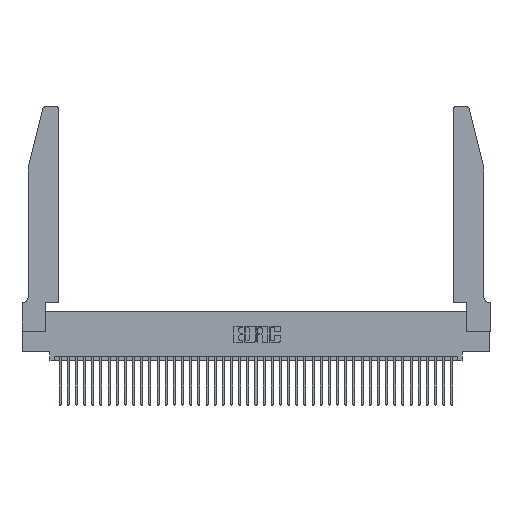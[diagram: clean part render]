
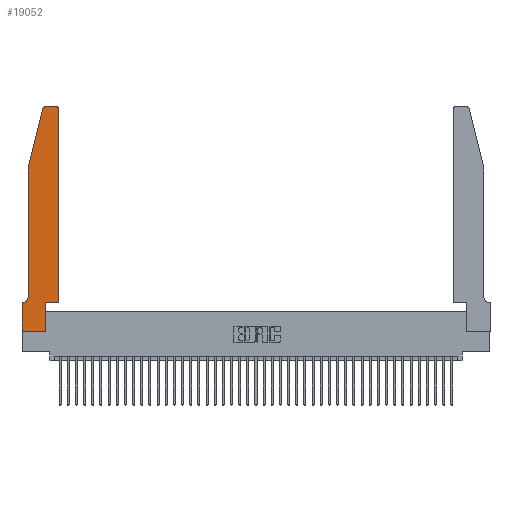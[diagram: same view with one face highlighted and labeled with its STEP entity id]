
A CAD part, top view. The second image highlights one B-rep face of the part: STEP entity #19052.
In plain terms, the highlighted planar face has unit normal (0, 0, 1).
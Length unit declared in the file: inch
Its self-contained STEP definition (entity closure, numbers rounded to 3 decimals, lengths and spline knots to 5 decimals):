
#363 = VECTOR ( 'NONE', #24415, 39.37008 ) ;
#1024 = AXIS2_PLACEMENT_3D ( 'NONE', #33563, #13965, #36864 ) ;
#1326 = VERTEX_POINT ( 'NONE', #29959 ) ;
#2813 = DIRECTION ( 'NONE',  ( 0., -1., 0. ) ) ;
#2863 = VECTOR ( 'NONE', #3584, 39.37008 ) ;
#3584 = DIRECTION ( 'NONE',  ( 1., 0., 0. ) ) ;
#4848 = CARTESIAN_POINT ( 'NONE',  ( 0.25487, 2.72718, 0.37 ) ) ;
#5324 = CIRCLE ( 'NONE', #18917, 0.03 ) ;
#5350 = LINE ( 'NONE', #19186, #13074 ) ;
#6082 = VERTEX_POINT ( 'NONE', #38138 ) ;
#6391 = PLANE ( 'NONE',  #8394 ) ;
#6947 = CIRCLE ( 'NONE', #11738, 0.07 ) ;
#7452 = VERTEX_POINT ( 'NONE', #22876 ) ;
#7635 = CARTESIAN_POINT ( 'NONE',  ( 0.4505, 0.35, 0.37 ) ) ;
#7849 = DIRECTION ( 'NONE',  ( 1., 0., 0. ) ) ;
#8078 = EDGE_CURVE ( 'NONE', #39810, #19090, #25536, .T. ) ;
#8394 = AXIS2_PLACEMENT_3D ( 'NONE', #29358, #42300, #32603 ) ;
#9282 = CARTESIAN_POINT ( 'NONE',  ( 0., 0.35, 0.37 ) ) ;
#10536 = CARTESIAN_POINT ( 'NONE',  ( 0., 0., 0.37 ) ) ;
#10678 = CARTESIAN_POINT ( 'NONE',  ( 0.284, 2.72, 0.37 ) ) ;
#11385 = CARTESIAN_POINT ( 'NONE',  ( 0.2865, 0.35, 0.37 ) ) ;
#11691 = ORIENTED_EDGE ( 'NONE', *, *, #30988, .T. ) ;
#11738 = AXIS2_PLACEMENT_3D ( 'NONE', #36510, #16945, #39782 ) ;
#11981 = CARTESIAN_POINT ( 'NONE',  ( 0.2605, 2.75, 0.37 ) ) ;
#12430 = ORIENTED_EDGE ( 'NONE', *, *, #36081, .T. ) ;
#13074 = VECTOR ( 'NONE', #2813, 39.37008 ) ;
#13147 = CARTESIAN_POINT ( 'NONE',  ( 0.2865, 0.35, 0.37 ) ) ;
#13965 = DIRECTION ( 'NONE',  ( 0., 0., 1. ) ) ;
#13988 = DIRECTION ( 'NONE',  ( 1., 0., 0. ) ) ;
#15048 = DIRECTION ( 'NONE',  ( -0.239, -0.971, 0. ) ) ;
#15246 = VECTOR ( 'NONE', #20415, 39.37008 ) ;
#15438 = VECTOR ( 'NONE', #25013, 39.37008 ) ;
#16472 = LINE ( 'NONE', #11981, #15438 ) ;
#16945 = DIRECTION ( 'NONE',  ( 0., 0., -1. ) ) ;
#16980 = EDGE_CURVE ( 'NONE', #7452, #6082, #5350, .T. ) ;
#17027 = EDGE_LOOP ( 'NONE', ( #11691, #37344, #27750, #29146, #17499, #17978, #35361, #12430, #35993, #18125, #27890, #22286 ) ) ;
#17499 = ORIENTED_EDGE ( 'NONE', *, *, #34721, .T. ) ;
#17978 = ORIENTED_EDGE ( 'NONE', *, *, #35241, .T. ) ;
#18125 = ORIENTED_EDGE ( 'NONE', *, *, #21626, .T. ) ;
#18326 = LINE ( 'NONE', #10536, #15246 ) ;
#18813 = EDGE_CURVE ( 'NONE', #36352, #7452, #26732, .T. ) ;
#18917 = AXIS2_PLACEMENT_3D ( 'NONE', #10678, #33585, #13988 ) ;
#19052 = ADVANCED_FACE ( 'NONE', ( #19534 ), #6391, .T. ) ;
#19090 = VERTEX_POINT ( 'NONE', #13147 ) ;
#19186 = CARTESIAN_POINT ( 'NONE',  ( 0.0755, 2., 0.37 ) ) ;
#19284 = CARTESIAN_POINT ( 'NONE',  ( 0.4205, 2.75, 0.37 ) ) ;
#19534 = FACE_OUTER_BOUND ( 'NONE', #17027, .T. ) ;
#20415 = DIRECTION ( 'NONE',  ( 0., -1., 0. ) ) ;
#21626 = EDGE_CURVE ( 'NONE', #19090, #39589, #35754, .T. ) ;
#22187 = EDGE_CURVE ( 'NONE', #1326, #37210, #32626, .T. ) ;
#22286 = ORIENTED_EDGE ( 'NONE', *, *, #22187, .T. ) ;
#22876 = CARTESIAN_POINT ( 'NONE',  ( 0.0755, 2., 0.37 ) ) ;
#24415 = DIRECTION ( 'NONE',  ( 0., 1., 0. ) ) ;
#25013 = DIRECTION ( 'NONE',  ( -1., 0., 0. ) ) ;
#25536 = LINE ( 'NONE', #11385, #363 ) ;
#25884 = CARTESIAN_POINT ( 'NONE',  ( 0.0755, 0.35, 0.37 ) ) ;
#25982 = CARTESIAN_POINT ( 'NONE',  ( 0., 0., 0.37 ) ) ;
#26484 = VERTEX_POINT ( 'NONE', #32318 ) ;
#26544 = CARTESIAN_POINT ( 'NONE',  ( 0., 0., 0.37 ) ) ;
#26732 = LINE ( 'NONE', #34632, #35424 ) ;
#27085 = VECTOR ( 'NONE', #7849, 39.37008 ) ;
#27470 = CARTESIAN_POINT ( 'NONE',  ( 0.4505, 0.35, 0.37 ) ) ;
#27526 = CARTESIAN_POINT ( 'NONE',  ( 0.2865, 0., 0.37 ) ) ;
#27540 = DIRECTION ( 'NONE',  ( 0., 1., 0. ) ) ;
#27750 = ORIENTED_EDGE ( 'NONE', *, *, #18813, .T. ) ;
#27890 = ORIENTED_EDGE ( 'NONE', *, *, #32850, .T. ) ;
#29146 = ORIENTED_EDGE ( 'NONE', *, *, #16980, .T. ) ;
#29210 = DIRECTION ( 'NONE',  ( -1., 0., 0. ) ) ;
#29358 = CARTESIAN_POINT ( 'NONE',  ( 0., 0.35, 0.37 ) ) ;
#29708 = CARTESIAN_POINT ( 'NONE',  ( 0.4505, 0.35, 0.37 ) ) ;
#29959 = CARTESIAN_POINT ( 'NONE',  ( 0.4505, 2.72, 0.37 ) ) ;
#30988 = EDGE_CURVE ( 'NONE', #37210, #26484, #16472, .T. ) ;
#31012 = VECTOR ( 'NONE', #29210, 39.37008 ) ;
#31095 = VERTEX_POINT ( 'NONE', #9282 ) ;
#32318 = CARTESIAN_POINT ( 'NONE',  ( 0.284, 2.75, 0.37 ) ) ;
#32603 = DIRECTION ( 'NONE',  ( 1., 0., 0. ) ) ;
#32626 = CIRCLE ( 'NONE', #1024, 0.03 ) ;
#32661 = VECTOR ( 'NONE', #27540, 39.37008 ) ;
#32850 = EDGE_CURVE ( 'NONE', #39589, #1326, #33695, .T. ) ;
#33563 = CARTESIAN_POINT ( 'NONE',  ( 0.4205, 2.72, 0.37 ) ) ;
#33585 = DIRECTION ( 'NONE',  ( 0., 0., 1. ) ) ;
#33695 = LINE ( 'NONE', #7635, #32661 ) ;
#34031 = EDGE_CURVE ( 'NONE', #31095, #40981, #18326, .T. ) ;
#34632 = CARTESIAN_POINT ( 'NONE',  ( 0.0755, 2., 0.37 ) ) ;
#34721 = EDGE_CURVE ( 'NONE', #6082, #35282, #6947, .T. ) ;
#35241 = EDGE_CURVE ( 'NONE', #35282, #31095, #39683, .T. ) ;
#35282 = VERTEX_POINT ( 'NONE', #39026 ) ;
#35361 = ORIENTED_EDGE ( 'NONE', *, *, #34031, .T. ) ;
#35424 = VECTOR ( 'NONE', #15048, 39.37008 ) ;
#35480 = EDGE_CURVE ( 'NONE', #26484, #36352, #5324, .T. ) ;
#35754 = LINE ( 'NONE', #27470, #27085 ) ;
#35993 = ORIENTED_EDGE ( 'NONE', *, *, #8078, .T. ) ;
#36081 = EDGE_CURVE ( 'NONE', #40981, #39810, #36716, .T. ) ;
#36352 = VERTEX_POINT ( 'NONE', #4848 ) ;
#36510 = CARTESIAN_POINT ( 'NONE',  ( 0.0055, 0.42, 0.37 ) ) ;
#36716 = LINE ( 'NONE', #26544, #2863 ) ;
#36864 = DIRECTION ( 'NONE',  ( 1., 0., 0. ) ) ;
#37210 = VERTEX_POINT ( 'NONE', #19284 ) ;
#37344 = ORIENTED_EDGE ( 'NONE', *, *, #35480, .T. ) ;
#38138 = CARTESIAN_POINT ( 'NONE',  ( 0.0755, 0.42, 0.37 ) ) ;
#39026 = CARTESIAN_POINT ( 'NONE',  ( 0.0055, 0.35, 0.37 ) ) ;
#39589 = VERTEX_POINT ( 'NONE', #29708 ) ;
#39683 = LINE ( 'NONE', #25884, #31012 ) ;
#39782 = DIRECTION ( 'NONE',  ( -1., 0., 0. ) ) ;
#39810 = VERTEX_POINT ( 'NONE', #27526 ) ;
#40981 = VERTEX_POINT ( 'NONE', #25982 ) ;
#42300 = DIRECTION ( 'NONE',  ( 0., 0., 1. ) ) ;
